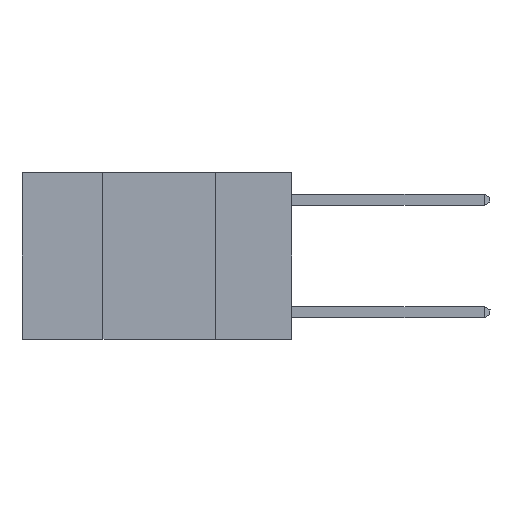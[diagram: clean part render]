
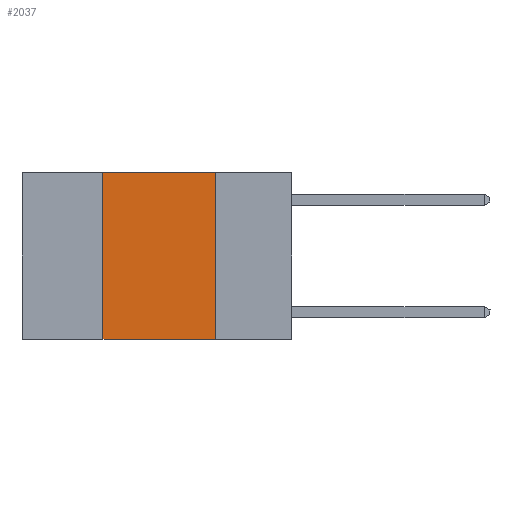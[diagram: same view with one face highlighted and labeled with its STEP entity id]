
A CAD part, left-side view. The second image highlights one B-rep face of the part: STEP entity #2037.
In plain terms, the highlighted planar face has unit normal (-1, 0, 0).
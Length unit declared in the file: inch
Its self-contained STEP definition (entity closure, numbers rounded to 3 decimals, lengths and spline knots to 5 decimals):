
#49 = CARTESIAN_POINT ( 'NONE',  ( 0., 0.17, 0. ) ) ;
#294 = VECTOR ( 'NONE', #6041, 39.37008 ) ;
#436 = ORIENTED_EDGE ( 'NONE', *, *, #1530, .F. ) ;
#859 = FACE_OUTER_BOUND ( 'NONE', #4929, .T. ) ;
#873 = VECTOR ( 'NONE', #6737, 39.37008 ) ;
#984 = VECTOR ( 'NONE', #4996, 39.37008 ) ;
#1530 = EDGE_CURVE ( 'NONE', #1892, #12199, #8968, .T. ) ;
#1892 = VERTEX_POINT ( 'NONE', #11641 ) ;
#2037 = ADVANCED_FACE ( 'NONE', ( #859 ), #8772, .F. ) ;
#3578 = EDGE_CURVE ( 'NONE', #1892, #8801, #9129, .T. ) ;
#3803 = VERTEX_POINT ( 'NONE', #5675 ) ;
#4929 = EDGE_LOOP ( 'NONE', ( #11860, #10758, #436, #11070 ) ) ;
#4996 = DIRECTION ( 'NONE',  ( 0., 0., -1. ) ) ;
#5042 = DIRECTION ( 'NONE',  ( 1., 0., 0. ) ) ;
#5470 = CARTESIAN_POINT ( 'NONE',  ( 0., 0.42, 0. ) ) ;
#5675 = CARTESIAN_POINT ( 'NONE',  ( 0., 0.17, 0. ) ) ;
#6041 = DIRECTION ( 'NONE',  ( 0., -1., 0. ) ) ;
#6185 = EDGE_CURVE ( 'NONE', #3803, #8801, #10995, .T. ) ;
#6612 = VECTOR ( 'NONE', #8167, 39.37008 ) ;
#6737 = DIRECTION ( 'NONE',  ( 0., 0., 1. ) ) ;
#7224 = CARTESIAN_POINT ( 'NONE',  ( 0., 0.6, -0.37 ) ) ;
#7558 = CARTESIAN_POINT ( 'NONE',  ( 0., 0.42, 0. ) ) ;
#7831 = LINE ( 'NONE', #11725, #294 ) ;
#8158 = DIRECTION ( 'NONE',  ( 0., 0., -1. ) ) ;
#8167 = DIRECTION ( 'NONE',  ( 0., -1., 0. ) ) ;
#8772 = PLANE ( 'NONE',  #8864 ) ;
#8801 = VERTEX_POINT ( 'NONE', #9020 ) ;
#8864 = AXIS2_PLACEMENT_3D ( 'NONE', #9006, #5042, #8158 ) ;
#8968 = LINE ( 'NONE', #7558, #873 ) ;
#9006 = CARTESIAN_POINT ( 'NONE',  ( 0., 0.6, 0. ) ) ;
#9020 = CARTESIAN_POINT ( 'NONE',  ( 0., 0.17, -0.37 ) ) ;
#9129 = LINE ( 'NONE', #7224, #6612 ) ;
#10758 = ORIENTED_EDGE ( 'NONE', *, *, #11023, .F. ) ;
#10995 = LINE ( 'NONE', #49, #984 ) ;
#11023 = EDGE_CURVE ( 'NONE', #12199, #3803, #7831, .T. ) ;
#11070 = ORIENTED_EDGE ( 'NONE', *, *, #3578, .T. ) ;
#11641 = CARTESIAN_POINT ( 'NONE',  ( 0., 0.42, -0.37 ) ) ;
#11725 = CARTESIAN_POINT ( 'NONE',  ( 0., 0.6, 0. ) ) ;
#11860 = ORIENTED_EDGE ( 'NONE', *, *, #6185, .F. ) ;
#12199 = VERTEX_POINT ( 'NONE', #5470 ) ;
